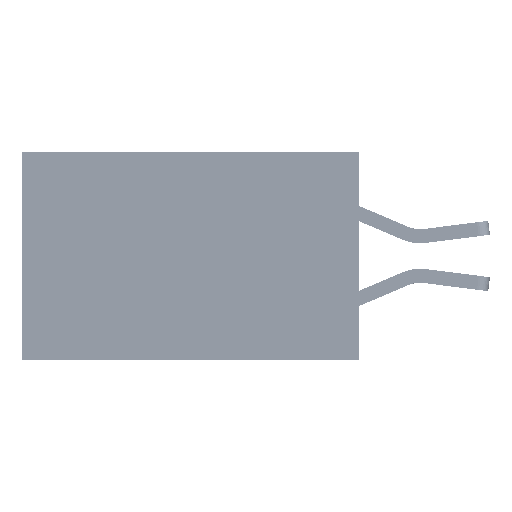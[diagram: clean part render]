
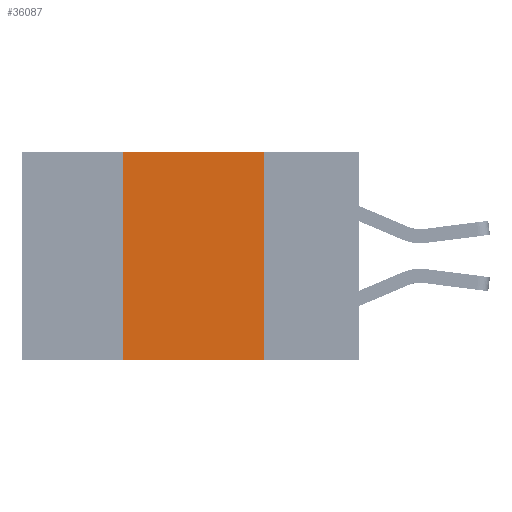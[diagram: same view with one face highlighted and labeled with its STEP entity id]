
A CAD part, left-side view. The second image highlights one B-rep face of the part: STEP entity #36087.
In plain terms, the highlighted planar face has unit normal (-1, 0, 0).
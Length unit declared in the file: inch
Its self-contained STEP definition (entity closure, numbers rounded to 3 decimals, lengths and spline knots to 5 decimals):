
#51 = DIRECTION ( 'NONE',  ( 0., 0., -1. ) ) ;
#330 = LINE ( 'NONE', #17804, #25844 ) ;
#2353 = DIRECTION ( 'NONE',  ( 0., 0., -1. ) ) ;
#2775 = CARTESIAN_POINT ( 'NONE',  ( 0., 0.42, 0. ) ) ;
#3888 = CARTESIAN_POINT ( 'NONE',  ( 0., 0.17, -0.37 ) ) ;
#4157 = VECTOR ( 'NONE', #30697, 39.37008 ) ;
#5076 = EDGE_CURVE ( 'NONE', #17984, #13526, #330, .T. ) ;
#6723 = PLANE ( 'NONE',  #27753 ) ;
#7637 = ORIENTED_EDGE ( 'NONE', *, *, #5076, .F. ) ;
#10846 = LINE ( 'NONE', #22716, #15042 ) ;
#11492 = ORIENTED_EDGE ( 'NONE', *, *, #24322, .T. ) ;
#13295 = VERTEX_POINT ( 'NONE', #3888 ) ;
#13526 = VERTEX_POINT ( 'NONE', #2775 ) ;
#14748 = FACE_OUTER_BOUND ( 'NONE', #39030, .T. ) ;
#15042 = VECTOR ( 'NONE', #22293, 39.37008 ) ;
#17804 = CARTESIAN_POINT ( 'NONE',  ( 0., 0.42, 0. ) ) ;
#17984 = VERTEX_POINT ( 'NONE', #32567 ) ;
#19325 = CARTESIAN_POINT ( 'NONE',  ( 0., 0.17, 0. ) ) ;
#20096 = CARTESIAN_POINT ( 'NONE',  ( 0., 0.6, 0. ) ) ;
#20858 = LINE ( 'NONE', #19325, #23986 ) ;
#21835 = LINE ( 'NONE', #41359, #4157 ) ;
#22293 = DIRECTION ( 'NONE',  ( 0., -1., 0. ) ) ;
#22716 = CARTESIAN_POINT ( 'NONE',  ( 0., 0.6, 0. ) ) ;
#23986 = VECTOR ( 'NONE', #2353, 39.37008 ) ;
#24322 = EDGE_CURVE ( 'NONE', #17984, #13295, #21835, .T. ) ;
#25844 = VECTOR ( 'NONE', #41559, 39.37008 ) ;
#27753 = AXIS2_PLACEMENT_3D ( 'NONE', #20096, #39631, #51 ) ;
#27777 = VERTEX_POINT ( 'NONE', #39214 ) ;
#28299 = EDGE_CURVE ( 'NONE', #13526, #27777, #10846, .T. ) ;
#30697 = DIRECTION ( 'NONE',  ( 0., -1., 0. ) ) ;
#32567 = CARTESIAN_POINT ( 'NONE',  ( 0., 0.42, -0.37 ) ) ;
#32881 = EDGE_CURVE ( 'NONE', #27777, #13295, #20858, .T. ) ;
#32892 = ORIENTED_EDGE ( 'NONE', *, *, #32881, .F. ) ;
#35245 = ORIENTED_EDGE ( 'NONE', *, *, #28299, .F. ) ;
#36087 = ADVANCED_FACE ( 'NONE', ( #14748 ), #6723, .F. ) ;
#39030 = EDGE_LOOP ( 'NONE', ( #32892, #35245, #7637, #11492 ) ) ;
#39214 = CARTESIAN_POINT ( 'NONE',  ( 0., 0.17, 0. ) ) ;
#39631 = DIRECTION ( 'NONE',  ( 1., 0., 0. ) ) ;
#41359 = CARTESIAN_POINT ( 'NONE',  ( 0., 0.6, -0.37 ) ) ;
#41559 = DIRECTION ( 'NONE',  ( 0., 0., 1. ) ) ;
